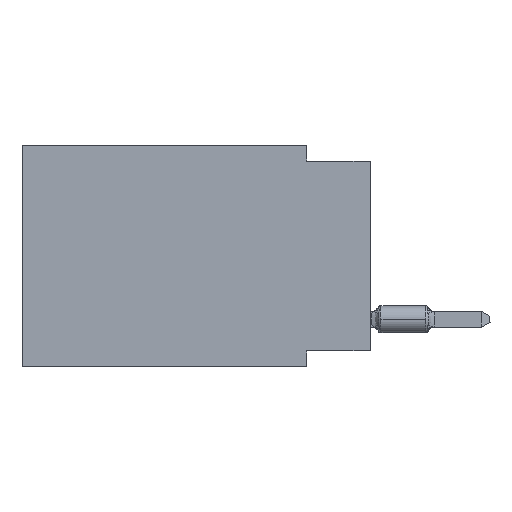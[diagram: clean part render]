
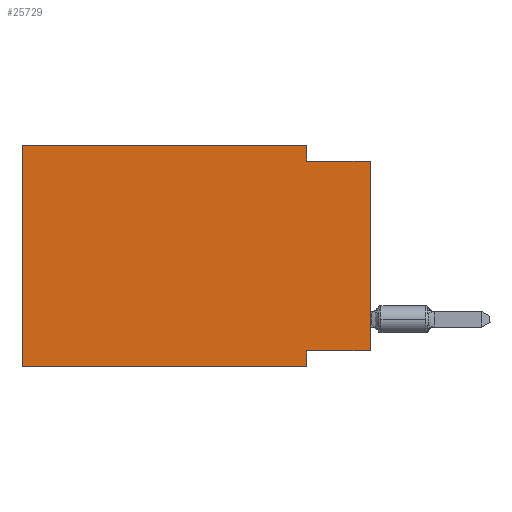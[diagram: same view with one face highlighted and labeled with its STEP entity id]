
A CAD part, left-side view. The second image highlights one B-rep face of the part: STEP entity #25729.
In plain terms, the highlighted planar face has unit normal (-1, 0, 0).
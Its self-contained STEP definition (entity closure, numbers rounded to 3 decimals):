
#983 = CARTESIAN_POINT ( 'NONE',  ( 0., 13.97, -8.89 ) ) ;
#1468 = VECTOR ( 'NONE', #15280, 1000. ) ;
#1947 = DIRECTION ( 'NONE',  ( 0., -1., 0. ) ) ;
#2823 = DIRECTION ( 'NONE',  ( 0., 0., 1. ) ) ;
#3853 = EDGE_CURVE ( 'NONE', #51155, #60872, #48045, .T. ) ;
#3946 = VECTOR ( 'NONE', #10042, 1000. ) ;
#4607 = CARTESIAN_POINT ( 'NONE',  ( 0., 2.54, -8.255 ) ) ;
#4764 = VERTEX_POINT ( 'NONE', #52265 ) ;
#5368 = CARTESIAN_POINT ( 'NONE',  ( 0., 13.97, 0. ) ) ;
#8049 = CARTESIAN_POINT ( 'NONE',  ( 0., 2.54, 0. ) ) ;
#8342 = EDGE_CURVE ( 'NONE', #60872, #58310, #31501, .T. ) ;
#9824 = VERTEX_POINT ( 'NONE', #54677 ) ;
#9911 = VECTOR ( 'NONE', #20222, 1000. ) ;
#10042 = DIRECTION ( 'NONE',  ( 0., -1., 0. ) ) ;
#10998 = ORIENTED_EDGE ( 'NONE', *, *, #8342, .F. ) ;
#11988 = ORIENTED_EDGE ( 'NONE', *, *, #33269, .T. ) ;
#12168 = DIRECTION ( 'NONE',  ( 0., -1., 0. ) ) ;
#12270 = CARTESIAN_POINT ( 'NONE',  ( 0., 2.54, -8.89 ) ) ;
#13747 = AXIS2_PLACEMENT_3D ( 'NONE', #30682, #35574, #50562 ) ;
#14117 = CARTESIAN_POINT ( 'NONE',  ( 0., 0., -8.255 ) ) ;
#14425 = ORIENTED_EDGE ( 'NONE', *, *, #24333, .T. ) ;
#15280 = DIRECTION ( 'NONE',  ( 0., 0., 1. ) ) ;
#15806 = EDGE_LOOP ( 'NONE', ( #11988, #48118, #35714, #55893, #62230, #14425, #10998, #55087 ) ) ;
#16235 = CARTESIAN_POINT ( 'NONE',  ( 0., 13.97, 0. ) ) ;
#17418 = CARTESIAN_POINT ( 'NONE',  ( 0., 13.97, 0. ) ) ;
#18331 = CARTESIAN_POINT ( 'NONE',  ( 0., 0., -0.635 ) ) ;
#20222 = DIRECTION ( 'NONE',  ( 0., 0., -1. ) ) ;
#24333 = EDGE_CURVE ( 'NONE', #9824, #58310, #30030, .T. ) ;
#25396 = VERTEX_POINT ( 'NONE', #18331 ) ;
#25729 = ADVANCED_FACE ( 'NONE', ( #45361 ), #60335, .F. ) ;
#27057 = VECTOR ( 'NONE', #38277, 1000. ) ;
#27393 = CARTESIAN_POINT ( 'NONE',  ( 0., 0., -8.255 ) ) ;
#28559 = DIRECTION ( 'NONE',  ( 0., 0., -1. ) ) ;
#30030 = LINE ( 'NONE', #983, #40095 ) ;
#30682 = CARTESIAN_POINT ( 'NONE',  ( 0., 13.97, 0. ) ) ;
#31501 = LINE ( 'NONE', #12270, #9911 ) ;
#32365 = CARTESIAN_POINT ( 'NONE',  ( 0., 0., -0.635 ) ) ;
#33269 = EDGE_CURVE ( 'NONE', #51155, #25396, #48447, .T. ) ;
#34632 = CARTESIAN_POINT ( 'NONE',  ( 0., 2.54, -8.89 ) ) ;
#35574 = DIRECTION ( 'NONE',  ( 1., 0., 0. ) ) ;
#35714 = ORIENTED_EDGE ( 'NONE', *, *, #47403, .F. ) ;
#38038 = LINE ( 'NONE', #8049, #39807 ) ;
#38277 = DIRECTION ( 'NONE',  ( 0., 1., 0. ) ) ;
#39807 = VECTOR ( 'NONE', #28559, 1000. ) ;
#40095 = VECTOR ( 'NONE', #1947, 1000. ) ;
#40973 = CARTESIAN_POINT ( 'NONE',  ( 0., 2.54, 0. ) ) ;
#41015 = LINE ( 'NONE', #16235, #1468 ) ;
#41238 = VECTOR ( 'NONE', #12168, 1000. ) ;
#41374 = VECTOR ( 'NONE', #2823, 1000. ) ;
#45361 = FACE_OUTER_BOUND ( 'NONE', #15806, .T. ) ;
#47403 = EDGE_CURVE ( 'NONE', #57571, #4764, #38038, .T. ) ;
#48045 = LINE ( 'NONE', #14117, #27057 ) ;
#48118 = ORIENTED_EDGE ( 'NONE', *, *, #55295, .F. ) ;
#48447 = LINE ( 'NONE', #62151, #41374 ) ;
#50562 = DIRECTION ( 'NONE',  ( 0., 0., -1. ) ) ;
#51155 = VERTEX_POINT ( 'NONE', #27393 ) ;
#52265 = CARTESIAN_POINT ( 'NONE',  ( 0., 2.54, -0.635 ) ) ;
#54235 = EDGE_CURVE ( 'NONE', #57899, #57571, #62051, .T. ) ;
#54677 = CARTESIAN_POINT ( 'NONE',  ( 0., 13.97, -8.89 ) ) ;
#55087 = ORIENTED_EDGE ( 'NONE', *, *, #3853, .F. ) ;
#55295 = EDGE_CURVE ( 'NONE', #4764, #25396, #62332, .T. ) ;
#55893 = ORIENTED_EDGE ( 'NONE', *, *, #54235, .F. ) ;
#57571 = VERTEX_POINT ( 'NONE', #40973 ) ;
#57899 = VERTEX_POINT ( 'NONE', #5368 ) ;
#58310 = VERTEX_POINT ( 'NONE', #34632 ) ;
#60335 = PLANE ( 'NONE',  #13747 ) ;
#60872 = VERTEX_POINT ( 'NONE', #4607 ) ;
#62051 = LINE ( 'NONE', #17418, #3946 ) ;
#62151 = CARTESIAN_POINT ( 'NONE',  ( 0., 0., 0. ) ) ;
#62230 = ORIENTED_EDGE ( 'NONE', *, *, #62830, .F. ) ;
#62332 = LINE ( 'NONE', #32365, #41238 ) ;
#62830 = EDGE_CURVE ( 'NONE', #9824, #57899, #41015, .T. ) ;
